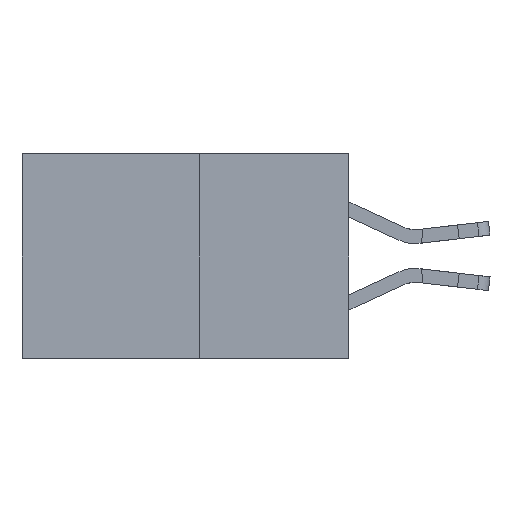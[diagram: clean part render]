
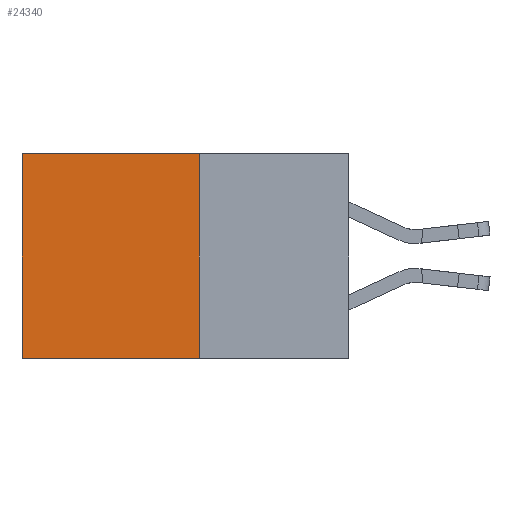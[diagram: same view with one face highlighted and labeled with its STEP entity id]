
A CAD part, left-side view. The second image highlights one B-rep face of the part: STEP entity #24340.
In plain terms, the highlighted planar face has unit normal (-1, 0, 0).
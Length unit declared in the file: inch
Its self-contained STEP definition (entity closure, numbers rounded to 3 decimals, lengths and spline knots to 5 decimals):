
#360 = DIRECTION ( 'NONE',  ( 0., 0., -1. ) ) ;
#492 = DIRECTION ( 'NONE',  ( 0., 0., -1. ) ) ;
#934 = VERTEX_POINT ( 'NONE', #8692 ) ;
#960 = DIRECTION ( 'NONE',  ( 0., 1., 0. ) ) ;
#1509 = LINE ( 'NONE', #24910, #11715 ) ;
#1778 = ORIENTED_EDGE ( 'NONE', *, *, #9608, .T. ) ;
#2007 = CARTESIAN_POINT ( 'NONE',  ( 0.277, 0.59, -0.37 ) ) ;
#2337 = ORIENTED_EDGE ( 'NONE', *, *, #19961, .F. ) ;
#3084 = VECTOR ( 'NONE', #14528, 39.37008 ) ;
#3632 = EDGE_CURVE ( 'NONE', #22759, #8679, #17752, .T. ) ;
#4362 = CARTESIAN_POINT ( 'NONE',  ( 0.277, 0.27, -0.37 ) ) ;
#8257 = VERTEX_POINT ( 'NONE', #9823 ) ;
#8679 = VERTEX_POINT ( 'NONE', #2007 ) ;
#8692 = CARTESIAN_POINT ( 'NONE',  ( 0.277, 0.59, 0. ) ) ;
#9264 = FACE_OUTER_BOUND ( 'NONE', #23537, .T. ) ;
#9608 = EDGE_CURVE ( 'NONE', #8257, #934, #13537, .T. ) ;
#9823 = CARTESIAN_POINT ( 'NONE',  ( 0.277, 0.27, 0. ) ) ;
#11053 = CARTESIAN_POINT ( 'NONE',  ( 0.277, 0.27, 0. ) ) ;
#11715 = VECTOR ( 'NONE', #492, 39.37008 ) ;
#12581 = DIRECTION ( 'NONE',  ( 1., 0., 0. ) ) ;
#12709 = ORIENTED_EDGE ( 'NONE', *, *, #13221, .T. ) ;
#13221 = EDGE_CURVE ( 'NONE', #934, #8679, #1509, .T. ) ;
#13537 = LINE ( 'NONE', #11053, #14180 ) ;
#14180 = VECTOR ( 'NONE', #25313, 39.37008 ) ;
#14528 = DIRECTION ( 'NONE',  ( 0., 0., -1. ) ) ;
#15235 = CARTESIAN_POINT ( 'NONE',  ( 0.277, 0.27, -0.37 ) ) ;
#16612 = PLANE ( 'NONE',  #25520 ) ;
#17106 = VECTOR ( 'NONE', #960, 39.37008 ) ;
#17752 = LINE ( 'NONE', #15235, #17106 ) ;
#19460 = ORIENTED_EDGE ( 'NONE', *, *, #3632, .F. ) ;
#19961 = EDGE_CURVE ( 'NONE', #8257, #22759, #24136, .T. ) ;
#22401 = CARTESIAN_POINT ( 'NONE',  ( 0.277, 0.27, -0.37 ) ) ;
#22759 = VERTEX_POINT ( 'NONE', #22401 ) ;
#23537 = EDGE_LOOP ( 'NONE', ( #12709, #19460, #2337, #1778 ) ) ;
#24136 = LINE ( 'NONE', #4362, #3084 ) ;
#24340 = ADVANCED_FACE ( 'NONE', ( #9264 ), #16612, .F. ) ;
#24775 = CARTESIAN_POINT ( 'NONE',  ( 0.277, 0.27, -0.37 ) ) ;
#24910 = CARTESIAN_POINT ( 'NONE',  ( 0.277, 0.59, -0.37 ) ) ;
#25313 = DIRECTION ( 'NONE',  ( 0., 1., 0. ) ) ;
#25520 = AXIS2_PLACEMENT_3D ( 'NONE', #24775, #12581, #360 ) ;
